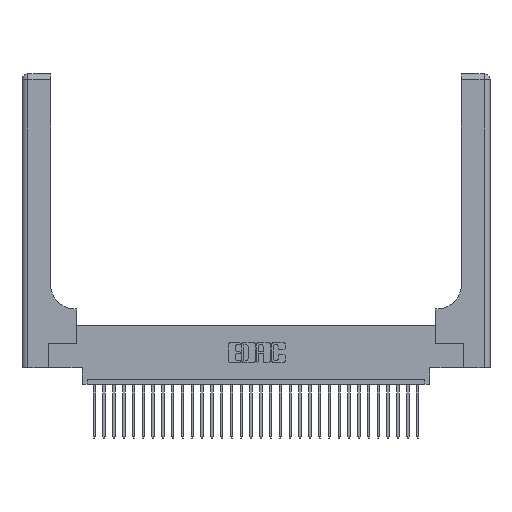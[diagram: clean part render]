
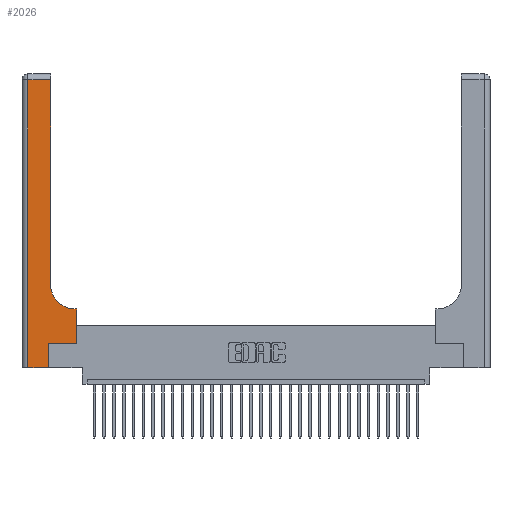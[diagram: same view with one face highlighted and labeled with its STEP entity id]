
A CAD part, top view. The second image highlights one B-rep face of the part: STEP entity #2026.
In plain terms, the highlighted planar face has unit normal (0, 0, 1).
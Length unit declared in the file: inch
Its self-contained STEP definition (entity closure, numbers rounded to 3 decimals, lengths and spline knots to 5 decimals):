
#125 = DIRECTION ( 'NONE',  ( 0., 1., 0. ) ) ;
#673 = CARTESIAN_POINT ( 'NONE',  ( 0.5585, 0.25, 0.37 ) ) ;
#883 = DIRECTION ( 'NONE',  ( -1., 0., 0. ) ) ;
#978 = DIRECTION ( 'NONE',  ( 0., 1., 0. ) ) ;
#1228 = CARTESIAN_POINT ( 'NONE',  ( 0., 2.94, 0.37 ) ) ;
#1230 = EDGE_CURVE ( 'NONE', #24241, #26181, #2801, .T. ) ;
#1441 = DIRECTION ( 'NONE',  ( -1., 0., 0. ) ) ;
#1947 = VERTEX_POINT ( 'NONE', #30252 ) ;
#2026 = ADVANCED_FACE ( 'NONE', ( #22847 ), #20519, .F. ) ;
#2801 = LINE ( 'NONE', #15035, #22099 ) ;
#2813 = DIRECTION ( 'NONE',  ( 1., 0., 0. ) ) ;
#3214 = VERTEX_POINT ( 'NONE', #11607 ) ;
#3362 = DIRECTION ( 'NONE',  ( 0., 0., -1. ) ) ;
#3720 = CARTESIAN_POINT ( 'NONE',  ( 0.5585, 0.6, 0.37 ) ) ;
#3819 = ORIENTED_EDGE ( 'NONE', *, *, #21648, .T. ) ;
#3913 = LINE ( 'NONE', #6711, #17444 ) ;
#5316 = VERTEX_POINT ( 'NONE', #10175 ) ;
#6570 = VERTEX_POINT ( 'NONE', #31395 ) ;
#6572 = LINE ( 'NONE', #7418, #16592 ) ;
#6711 = CARTESIAN_POINT ( 'NONE',  ( 0.269, 0., 0.37 ) ) ;
#7317 = VECTOR ( 'NONE', #21033, 39.37008 ) ;
#7418 = CARTESIAN_POINT ( 'NONE',  ( 0.2915, 3., 0.37 ) ) ;
#7448 = AXIS2_PLACEMENT_3D ( 'NONE', #25703, #3362, #20729 ) ;
#7643 = DIRECTION ( 'NONE',  ( 1., 0., 0. ) ) ;
#7869 = LINE ( 'NONE', #673, #26468 ) ;
#9318 = EDGE_LOOP ( 'NONE', ( #29454, #3819, #10861, #13494, #20601, #9941, #12701, #28905, #18440 ) ) ;
#9941 = ORIENTED_EDGE ( 'NONE', *, *, #22610, .T. ) ;
#10124 = CARTESIAN_POINT ( 'NONE',  ( 0.269, 0.25, 0.37 ) ) ;
#10175 = CARTESIAN_POINT ( 'NONE',  ( 0.2915, 0.85, 0.37 ) ) ;
#10343 = EDGE_CURVE ( 'NONE', #5316, #6570, #6572, .T. ) ;
#10861 = ORIENTED_EDGE ( 'NONE', *, *, #25996, .T. ) ;
#11047 = CARTESIAN_POINT ( 'NONE',  ( 0.06, 3., 0.37 ) ) ;
#11589 = CARTESIAN_POINT ( 'NONE',  ( 0.5585, 0.25, 0.37 ) ) ;
#11607 = CARTESIAN_POINT ( 'NONE',  ( 0.06, 2.94, 0.37 ) ) ;
#12701 = ORIENTED_EDGE ( 'NONE', *, *, #12931, .T. ) ;
#12931 = EDGE_CURVE ( 'NONE', #26180, #24002, #7869, .T. ) ;
#13494 = ORIENTED_EDGE ( 'NONE', *, *, #1230, .T. ) ;
#13651 = VERTEX_POINT ( 'NONE', #30412 ) ;
#15035 = CARTESIAN_POINT ( 'NONE',  ( 0., 0., 0.37 ) ) ;
#15106 = VECTOR ( 'NONE', #24877, 39.37008 ) ;
#15604 = DIRECTION ( 'NONE',  ( 0., 0., -1. ) ) ;
#16008 = LINE ( 'NONE', #1228, #21902 ) ;
#16592 = VECTOR ( 'NONE', #125, 39.37008 ) ;
#16706 = AXIS2_PLACEMENT_3D ( 'NONE', #25495, #15604, #883 ) ;
#17444 = VECTOR ( 'NONE', #29735, 39.37008 ) ;
#17625 = EDGE_CURVE ( 'NONE', #24002, #1947, #20575, .T. ) ;
#17695 = VECTOR ( 'NONE', #7643, 39.37008 ) ;
#18440 = ORIENTED_EDGE ( 'NONE', *, *, #23338, .T. ) ;
#18556 = CARTESIAN_POINT ( 'NONE',  ( 0.06, 0., 0.37 ) ) ;
#20519 = PLANE ( 'NONE',  #16706 ) ;
#20575 = LINE ( 'NONE', #27142, #15106 ) ;
#20601 = ORIENTED_EDGE ( 'NONE', *, *, #20730, .T. ) ;
#20729 = DIRECTION ( 'NONE',  ( 1., 0., 0. ) ) ;
#20730 = EDGE_CURVE ( 'NONE', #26181, #13651, #3913, .T. ) ;
#21033 = DIRECTION ( 'NONE',  ( 0., -1., 0. ) ) ;
#21648 = EDGE_CURVE ( 'NONE', #6570, #3214, #16008, .T. ) ;
#21902 = VECTOR ( 'NONE', #1441, 39.37008 ) ;
#22099 = VECTOR ( 'NONE', #2813, 39.37008 ) ;
#22610 = EDGE_CURVE ( 'NONE', #13651, #26180, #31654, .T. ) ;
#22847 = FACE_OUTER_BOUND ( 'NONE', #9318, .T. ) ;
#23338 = EDGE_CURVE ( 'NONE', #1947, #5316, #30059, .T. ) ;
#24002 = VERTEX_POINT ( 'NONE', #3720 ) ;
#24181 = CARTESIAN_POINT ( 'NONE',  ( 0.269, 0., 0.37 ) ) ;
#24241 = VERTEX_POINT ( 'NONE', #18556 ) ;
#24877 = DIRECTION ( 'NONE',  ( -1., 0., 0. ) ) ;
#25495 = CARTESIAN_POINT ( 'NONE',  ( 0., 3., 0.37 ) ) ;
#25703 = CARTESIAN_POINT ( 'NONE',  ( 0.5415, 0.85, 0.37 ) ) ;
#25996 = EDGE_CURVE ( 'NONE', #3214, #24241, #26671, .T. ) ;
#26180 = VERTEX_POINT ( 'NONE', #11589 ) ;
#26181 = VERTEX_POINT ( 'NONE', #24181 ) ;
#26468 = VECTOR ( 'NONE', #978, 39.37008 ) ;
#26671 = LINE ( 'NONE', #11047, #7317 ) ;
#27142 = CARTESIAN_POINT ( 'NONE',  ( 0.2915, 0.6, 0.37 ) ) ;
#28905 = ORIENTED_EDGE ( 'NONE', *, *, #17625, .T. ) ;
#29454 = ORIENTED_EDGE ( 'NONE', *, *, #10343, .T. ) ;
#29735 = DIRECTION ( 'NONE',  ( 0., 1., 0. ) ) ;
#30059 = CIRCLE ( 'NONE', #7448, 0.25 ) ;
#30252 = CARTESIAN_POINT ( 'NONE',  ( 0.5415, 0.6, 0.37 ) ) ;
#30412 = CARTESIAN_POINT ( 'NONE',  ( 0.269, 0.25, 0.37 ) ) ;
#31395 = CARTESIAN_POINT ( 'NONE',  ( 0.2915, 2.94, 0.37 ) ) ;
#31654 = LINE ( 'NONE', #10124, #17695 ) ;
